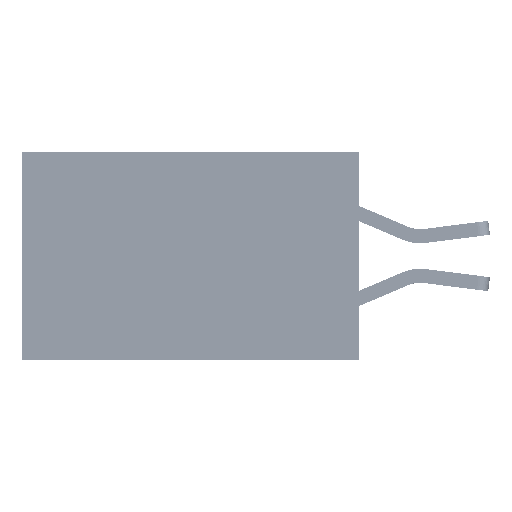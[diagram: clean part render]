
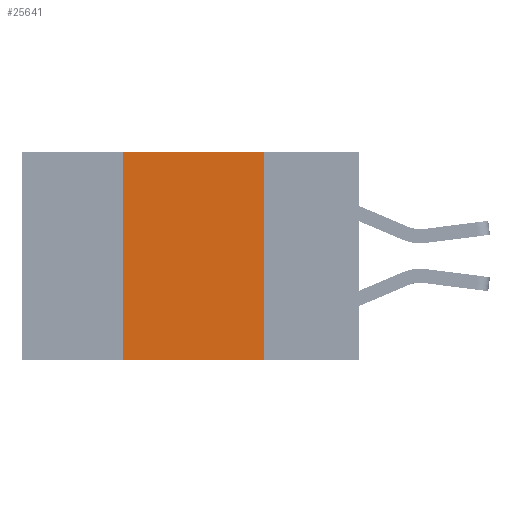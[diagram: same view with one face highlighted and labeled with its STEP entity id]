
A CAD part, left-side view. The second image highlights one B-rep face of the part: STEP entity #25641.
In plain terms, the highlighted planar face has unit normal (-1, 0, 0).
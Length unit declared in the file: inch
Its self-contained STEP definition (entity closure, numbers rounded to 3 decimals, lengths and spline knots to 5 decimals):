
#4211 = VECTOR ( 'NONE', #21152, 39.37008 ) ;
#4687 = CARTESIAN_POINT ( 'NONE',  ( 0., 0.6, 0. ) ) ;
#4953 = CARTESIAN_POINT ( 'NONE',  ( 0., 0.6, -0.37 ) ) ;
#5719 = CARTESIAN_POINT ( 'NONE',  ( 0., 0.17, -0.37 ) ) ;
#6454 = VERTEX_POINT ( 'NONE', #5719 ) ;
#7347 = VERTEX_POINT ( 'NONE', #30678 ) ;
#8245 = CARTESIAN_POINT ( 'NONE',  ( 0., 0.17, 0. ) ) ;
#8767 = LINE ( 'NONE', #4687, #11671 ) ;
#11671 = VECTOR ( 'NONE', #16895, 39.37008 ) ;
#13060 = LINE ( 'NONE', #4953, #17353 ) ;
#13804 = CARTESIAN_POINT ( 'NONE',  ( 0., 0.6, 0. ) ) ;
#14192 = DIRECTION ( 'NONE',  ( 0., 0., -1. ) ) ;
#14334 = VERTEX_POINT ( 'NONE', #27264 ) ;
#16714 = VERTEX_POINT ( 'NONE', #38555 ) ;
#16895 = DIRECTION ( 'NONE',  ( 0., -1., 0. ) ) ;
#16934 = CARTESIAN_POINT ( 'NONE',  ( 0., 0.42, 0. ) ) ;
#17253 = PLANE ( 'NONE',  #38163 ) ;
#17353 = VECTOR ( 'NONE', #25872, 39.37008 ) ;
#19504 = EDGE_LOOP ( 'NONE', ( #24634, #24024, #32202, #38552 ) ) ;
#20148 = DIRECTION ( 'NONE',  ( 1., 0., 0. ) ) ;
#21152 = DIRECTION ( 'NONE',  ( 0., 0., -1. ) ) ;
#22226 = EDGE_CURVE ( 'NONE', #16714, #7347, #34837, .T. ) ;
#24024 = ORIENTED_EDGE ( 'NONE', *, *, #30083, .F. ) ;
#24634 = ORIENTED_EDGE ( 'NONE', *, *, #28525, .F. ) ;
#25358 = VECTOR ( 'NONE', #26035, 39.37008 ) ;
#25641 = ADVANCED_FACE ( 'NONE', ( #28873 ), #17253, .F. ) ;
#25872 = DIRECTION ( 'NONE',  ( 0., -1., 0. ) ) ;
#26035 = DIRECTION ( 'NONE',  ( 0., 0., 1. ) ) ;
#27264 = CARTESIAN_POINT ( 'NONE',  ( 0., 0.17, 0. ) ) ;
#28525 = EDGE_CURVE ( 'NONE', #14334, #6454, #34084, .T. ) ;
#28873 = FACE_OUTER_BOUND ( 'NONE', #19504, .T. ) ;
#30083 = EDGE_CURVE ( 'NONE', #7347, #14334, #8767, .T. ) ;
#30178 = EDGE_CURVE ( 'NONE', #16714, #6454, #13060, .T. ) ;
#30678 = CARTESIAN_POINT ( 'NONE',  ( 0., 0.42, 0. ) ) ;
#32202 = ORIENTED_EDGE ( 'NONE', *, *, #22226, .F. ) ;
#34084 = LINE ( 'NONE', #8245, #4211 ) ;
#34837 = LINE ( 'NONE', #16934, #25358 ) ;
#38163 = AXIS2_PLACEMENT_3D ( 'NONE', #13804, #20148, #14192 ) ;
#38552 = ORIENTED_EDGE ( 'NONE', *, *, #30178, .T. ) ;
#38555 = CARTESIAN_POINT ( 'NONE',  ( 0., 0.42, -0.37 ) ) ;
